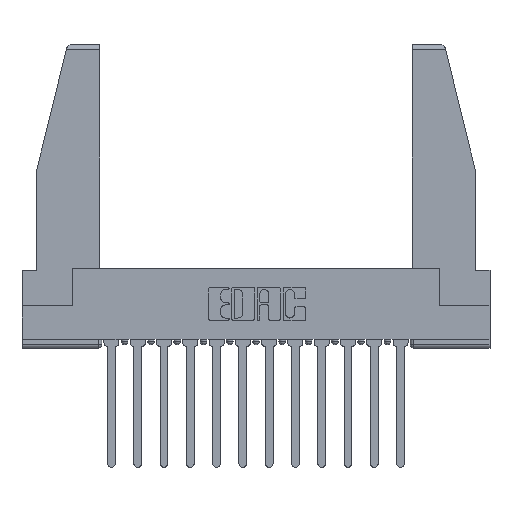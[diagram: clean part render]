
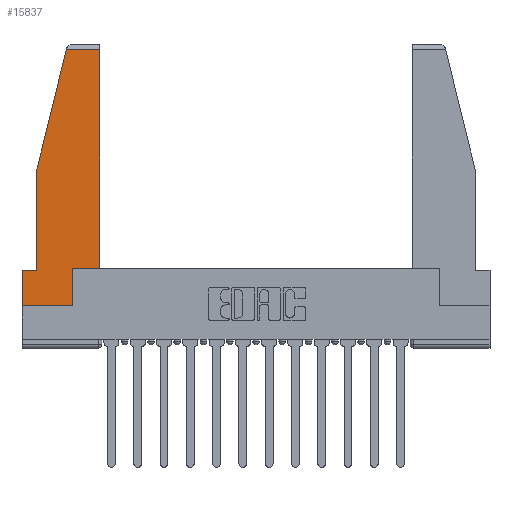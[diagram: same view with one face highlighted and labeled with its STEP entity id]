
A CAD part, top view. The second image highlights one B-rep face of the part: STEP entity #15837.
In plain terms, the highlighted planar face has unit normal (0, 0, 1).
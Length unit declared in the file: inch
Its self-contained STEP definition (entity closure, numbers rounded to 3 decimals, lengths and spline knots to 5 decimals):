
#278 = ORIENTED_EDGE ( 'NONE', *, *, #16153, .T. ) ;
#559 = VERTEX_POINT ( 'NONE', #10982 ) ;
#618 = ORIENTED_EDGE ( 'NONE', *, *, #3355, .T. ) ;
#919 = VERTEX_POINT ( 'NONE', #6709 ) ;
#1447 = ORIENTED_EDGE ( 'NONE', *, *, #5600, .T. ) ;
#1523 = DIRECTION ( 'NONE',  ( 1., 0., 0. ) ) ;
#2057 = VECTOR ( 'NONE', #9089, 39.37008 ) ;
#2367 = VERTEX_POINT ( 'NONE', #3384 ) ;
#2786 = CARTESIAN_POINT ( 'NONE',  ( 0., 0.21, 0. ) ) ;
#2861 = CARTESIAN_POINT ( 'NONE',  ( 0.297, 0.223, 0. ) ) ;
#2905 = VERTEX_POINT ( 'NONE', #5815 ) ;
#3171 = ORIENTED_EDGE ( 'NONE', *, *, #13881, .T. ) ;
#3355 = EDGE_CURVE ( 'NONE', #2905, #14414, #10051, .T. ) ;
#3384 = CARTESIAN_POINT ( 'NONE',  ( 0.297, 0., 0. ) ) ;
#3775 = DIRECTION ( 'NONE',  ( 1., 0., 0. ) ) ;
#4022 = PLANE ( 'NONE',  #4061 ) ;
#4061 = AXIS2_PLACEMENT_3D ( 'NONE', #11741, #12894, #1523 ) ;
#4275 = DIRECTION ( 'NONE',  ( -1., 0., 0. ) ) ;
#4735 = CARTESIAN_POINT ( 'NONE',  ( 0., 0.21, 0. ) ) ;
#4928 = LINE ( 'NONE', #9495, #15846 ) ;
#5025 = DIRECTION ( 'NONE',  ( -0.239, -0.971, 0. ) ) ;
#5092 = EDGE_CURVE ( 'NONE', #12700, #2905, #5813, .T. ) ;
#5117 = CARTESIAN_POINT ( 'NONE',  ( 0.297, 0.223, 0. ) ) ;
#5390 = LINE ( 'NONE', #9765, #7415 ) ;
#5600 = EDGE_CURVE ( 'NONE', #919, #2367, #4928, .T. ) ;
#5779 = DIRECTION ( 'NONE',  ( 0., -1., 0. ) ) ;
#5813 = LINE ( 'NONE', #13861, #8615 ) ;
#5815 = CARTESIAN_POINT ( 'NONE',  ( 0.086, 0.8, 0. ) ) ;
#6065 = LINE ( 'NONE', #5117, #13361 ) ;
#6109 = ORIENTED_EDGE ( 'NONE', *, *, #16385, .T. ) ;
#6660 = LINE ( 'NONE', #2786, #8837 ) ;
#6709 = CARTESIAN_POINT ( 'NONE',  ( 0., 0., 0. ) ) ;
#6994 = VECTOR ( 'NONE', #7856, 39.37008 ) ;
#7141 = CARTESIAN_POINT ( 'NONE',  ( 0.086, 0.8, 0. ) ) ;
#7415 = VECTOR ( 'NONE', #7539, 39.37008 ) ;
#7539 = DIRECTION ( 'NONE',  ( 0., 1., 0. ) ) ;
#7856 = DIRECTION ( 'NONE',  ( 0., -1., 0. ) ) ;
#7892 = LINE ( 'NONE', #9592, #8494 ) ;
#7975 = CARTESIAN_POINT ( 'NONE',  ( 0.297, 0., 0. ) ) ;
#8494 = VECTOR ( 'NONE', #4275, 39.37008 ) ;
#8615 = VECTOR ( 'NONE', #5025, 39.37008 ) ;
#8701 = ORIENTED_EDGE ( 'NONE', *, *, #12060, .T. ) ;
#8837 = VECTOR ( 'NONE', #11671, 39.37008 ) ;
#8981 = EDGE_CURVE ( 'NONE', #15368, #9367, #6065, .T. ) ;
#8985 = FACE_OUTER_BOUND ( 'NONE', #12481, .T. ) ;
#9089 = DIRECTION ( 'NONE',  ( 0., 1., 0. ) ) ;
#9250 = VECTOR ( 'NONE', #5779, 39.37008 ) ;
#9367 = VERTEX_POINT ( 'NONE', #14849 ) ;
#9495 = CARTESIAN_POINT ( 'NONE',  ( 0., 0., 0. ) ) ;
#9592 = CARTESIAN_POINT ( 'NONE',  ( 0., 1.52, 0. ) ) ;
#9765 = CARTESIAN_POINT ( 'NONE',  ( 0.461, 0.223, 0. ) ) ;
#9921 = VERTEX_POINT ( 'NONE', #4735 ) ;
#10051 = LINE ( 'NONE', #7141, #9250 ) ;
#10347 = CARTESIAN_POINT ( 'NONE',  ( 0., 0.21, 0. ) ) ;
#10982 = CARTESIAN_POINT ( 'NONE',  ( 0.461, 1.52, 0. ) ) ;
#11330 = ORIENTED_EDGE ( 'NONE', *, *, #5092, .T. ) ;
#11393 = CARTESIAN_POINT ( 'NONE',  ( 0.086, 0.21, 0. ) ) ;
#11533 = LINE ( 'NONE', #10347, #6994 ) ;
#11671 = DIRECTION ( 'NONE',  ( -1., 0., 0. ) ) ;
#11741 = CARTESIAN_POINT ( 'NONE',  ( 0., 0., 0. ) ) ;
#12060 = EDGE_CURVE ( 'NONE', #559, #12700, #7892, .T. ) ;
#12481 = EDGE_LOOP ( 'NONE', ( #278, #8701, #11330, #618, #12868, #6109, #1447, #3171, #16396 ) ) ;
#12700 = VERTEX_POINT ( 'NONE', #15414 ) ;
#12868 = ORIENTED_EDGE ( 'NONE', *, *, #13847, .T. ) ;
#12894 = DIRECTION ( 'NONE',  ( 0., 0., 1. ) ) ;
#13155 = LINE ( 'NONE', #7975, #2057 ) ;
#13361 = VECTOR ( 'NONE', #3775, 39.37008 ) ;
#13847 = EDGE_CURVE ( 'NONE', #14414, #9921, #6660, .T. ) ;
#13861 = CARTESIAN_POINT ( 'NONE',  ( 0.271, 1.55, 0. ) ) ;
#13881 = EDGE_CURVE ( 'NONE', #2367, #15368, #13155, .T. ) ;
#14414 = VERTEX_POINT ( 'NONE', #11393 ) ;
#14443 = DIRECTION ( 'NONE',  ( 1., 0., 0. ) ) ;
#14849 = CARTESIAN_POINT ( 'NONE',  ( 0.461, 0.223, 0. ) ) ;
#15368 = VERTEX_POINT ( 'NONE', #2861 ) ;
#15414 = CARTESIAN_POINT ( 'NONE',  ( 0.2636, 1.52, 0. ) ) ;
#15837 = ADVANCED_FACE ( 'NONE', ( #8985 ), #4022, .T. ) ;
#15846 = VECTOR ( 'NONE', #14443, 39.37008 ) ;
#16153 = EDGE_CURVE ( 'NONE', #9367, #559, #5390, .T. ) ;
#16385 = EDGE_CURVE ( 'NONE', #9921, #919, #11533, .T. ) ;
#16396 = ORIENTED_EDGE ( 'NONE', *, *, #8981, .T. ) ;
